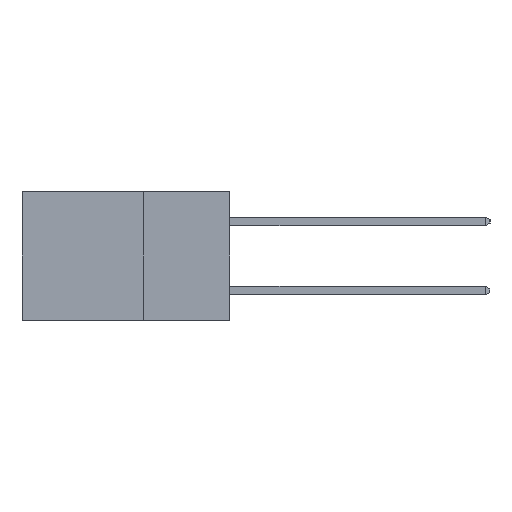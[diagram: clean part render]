
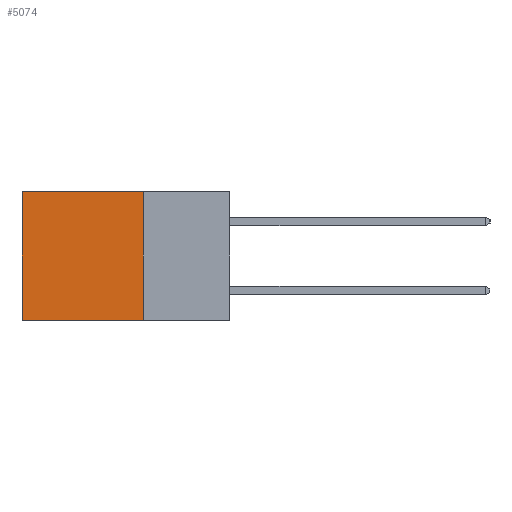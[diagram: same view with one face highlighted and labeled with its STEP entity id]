
A CAD part, left-side view. The second image highlights one B-rep face of the part: STEP entity #5074.
In plain terms, the highlighted planar face has unit normal (-1, 0, 0).
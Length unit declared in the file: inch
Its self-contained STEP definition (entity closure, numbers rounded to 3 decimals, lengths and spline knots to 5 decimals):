
#274 = EDGE_CURVE ( 'NONE', #10725, #622, #9861, .T. ) ;
#622 = VERTEX_POINT ( 'NONE', #5913 ) ;
#656 = CARTESIAN_POINT ( 'NONE',  ( 0.298, 0.25, 0. ) ) ;
#1310 = CARTESIAN_POINT ( 'NONE',  ( 0.298, 0.6, 0. ) ) ;
#1471 = DIRECTION ( 'NONE',  ( 0., 0., -1. ) ) ;
#1857 = CARTESIAN_POINT ( 'NONE',  ( 0.298, 0.25, 0. ) ) ;
#3321 = CARTESIAN_POINT ( 'NONE',  ( 0.298, 0.25, -0.37 ) ) ;
#3683 = CARTESIAN_POINT ( 'NONE',  ( 0.298, 0.6, -0.37 ) ) ;
#4463 = AXIS2_PLACEMENT_3D ( 'NONE', #1857, #7236, #1471 ) ;
#4535 = VECTOR ( 'NONE', #10245, 39.37008 ) ;
#4883 = LINE ( 'NONE', #8743, #7503 ) ;
#4911 = CARTESIAN_POINT ( 'NONE',  ( 0.298, 0.25, 0. ) ) ;
#5050 = EDGE_CURVE ( 'NONE', #10725, #12642, #4883, .T. ) ;
#5074 = ADVANCED_FACE ( 'NONE', ( #12110 ), #12169, .F. ) ;
#5472 = DIRECTION ( 'NONE',  ( 0., 1., 0. ) ) ;
#5913 = CARTESIAN_POINT ( 'NONE',  ( 0.298, 0.6, 0. ) ) ;
#6072 = LINE ( 'NONE', #3321, #8334 ) ;
#6313 = CARTESIAN_POINT ( 'NONE',  ( 0.298, 0.25, -0.37 ) ) ;
#6737 = EDGE_LOOP ( 'NONE', ( #11945, #10527, #10167, #11981 ) ) ;
#7124 = EDGE_CURVE ( 'NONE', #12642, #8895, #6072, .T. ) ;
#7149 = LINE ( 'NONE', #1310, #4535 ) ;
#7236 = DIRECTION ( 'NONE',  ( 1., 0., 0. ) ) ;
#7503 = VECTOR ( 'NONE', #12159, 39.37008 ) ;
#8334 = VECTOR ( 'NONE', #5472, 39.37008 ) ;
#8743 = CARTESIAN_POINT ( 'NONE',  ( 0.298, 0.25, 0. ) ) ;
#8895 = VERTEX_POINT ( 'NONE', #3683 ) ;
#9861 = LINE ( 'NONE', #4911, #12207 ) ;
#10167 = ORIENTED_EDGE ( 'NONE', *, *, #5050, .F. ) ;
#10245 = DIRECTION ( 'NONE',  ( 0., 0., -1. ) ) ;
#10433 = EDGE_CURVE ( 'NONE', #622, #8895, #7149, .T. ) ;
#10527 = ORIENTED_EDGE ( 'NONE', *, *, #7124, .F. ) ;
#10725 = VERTEX_POINT ( 'NONE', #656 ) ;
#11945 = ORIENTED_EDGE ( 'NONE', *, *, #10433, .T. ) ;
#11981 = ORIENTED_EDGE ( 'NONE', *, *, #274, .T. ) ;
#12110 = FACE_OUTER_BOUND ( 'NONE', #6737, .T. ) ;
#12159 = DIRECTION ( 'NONE',  ( 0., 0., -1. ) ) ;
#12169 = PLANE ( 'NONE',  #4463 ) ;
#12207 = VECTOR ( 'NONE', #12655, 39.37008 ) ;
#12642 = VERTEX_POINT ( 'NONE', #6313 ) ;
#12655 = DIRECTION ( 'NONE',  ( 0., 1., 0. ) ) ;
